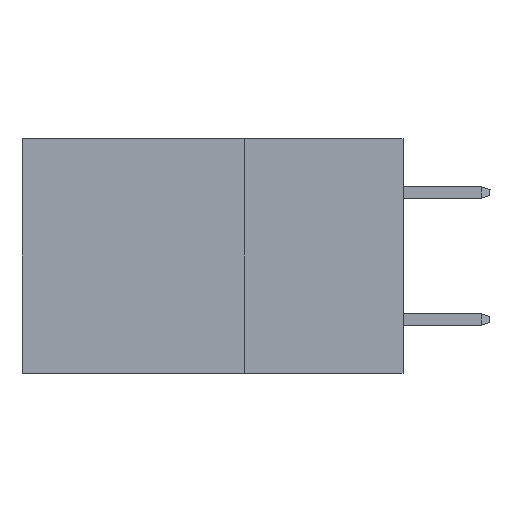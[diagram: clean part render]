
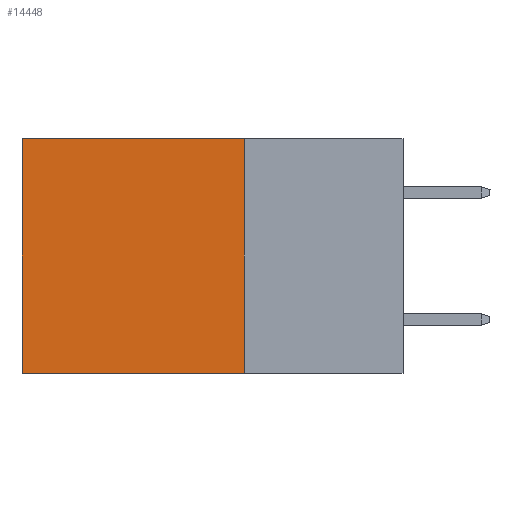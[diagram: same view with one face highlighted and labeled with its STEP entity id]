
A CAD part, left-side view. The second image highlights one B-rep face of the part: STEP entity #14448.
In plain terms, the highlighted planar face has unit normal (-1, 0, 0).
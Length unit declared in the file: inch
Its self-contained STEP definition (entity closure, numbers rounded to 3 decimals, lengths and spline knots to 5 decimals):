
#134 = DIRECTION ( 'NONE',  ( 0., 1., 0. ) ) ;
#319 = CARTESIAN_POINT ( 'NONE',  ( 0.2875, 0.6, 0. ) ) ;
#532 = PLANE ( 'NONE',  #3346 ) ;
#614 = FACE_OUTER_BOUND ( 'NONE', #8487, .T. ) ;
#944 = VERTEX_POINT ( 'NONE', #319 ) ;
#1567 = CARTESIAN_POINT ( 'NONE',  ( 0.2875, 0.25, 0. ) ) ;
#1646 = VERTEX_POINT ( 'NONE', #4934 ) ;
#2343 = EDGE_CURVE ( 'NONE', #9712, #6447, #3693, .T. ) ;
#2449 = ORIENTED_EDGE ( 'NONE', *, *, #6213, .T. ) ;
#2608 = CARTESIAN_POINT ( 'NONE',  ( 0.2875, 0.25, 0. ) ) ;
#3262 = VECTOR ( 'NONE', #4886, 39.37008 ) ;
#3346 = AXIS2_PLACEMENT_3D ( 'NONE', #14876, #4416, #5697 ) ;
#3693 = LINE ( 'NONE', #8888, #5870 ) ;
#4402 = EDGE_CURVE ( 'NONE', #944, #1646, #10922, .T. ) ;
#4416 = DIRECTION ( 'NONE',  ( 1., 0., 0. ) ) ;
#4886 = DIRECTION ( 'NONE',  ( 0., 1., 0. ) ) ;
#4934 = CARTESIAN_POINT ( 'NONE',  ( 0.2875, 0.6, -0.37 ) ) ;
#5075 = DIRECTION ( 'NONE',  ( 0., 0., -1. ) ) ;
#5697 = DIRECTION ( 'NONE',  ( 0., 0., -1. ) ) ;
#5870 = VECTOR ( 'NONE', #5075, 39.37008 ) ;
#5937 = VECTOR ( 'NONE', #134, 39.37008 ) ;
#6213 = EDGE_CURVE ( 'NONE', #9712, #944, #7868, .T. ) ;
#6447 = VERTEX_POINT ( 'NONE', #16330 ) ;
#7868 = LINE ( 'NONE', #1567, #5937 ) ;
#7979 = ORIENTED_EDGE ( 'NONE', *, *, #4402, .T. ) ;
#8185 = EDGE_CURVE ( 'NONE', #6447, #1646, #13883, .T. ) ;
#8441 = DIRECTION ( 'NONE',  ( 0., 0., -1. ) ) ;
#8487 = EDGE_LOOP ( 'NONE', ( #7979, #9019, #13822, #2449 ) ) ;
#8888 = CARTESIAN_POINT ( 'NONE',  ( 0.2875, 0.25, 0. ) ) ;
#9019 = ORIENTED_EDGE ( 'NONE', *, *, #8185, .F. ) ;
#9712 = VERTEX_POINT ( 'NONE', #2608 ) ;
#10922 = LINE ( 'NONE', #16016, #13524 ) ;
#13524 = VECTOR ( 'NONE', #8441, 39.37008 ) ;
#13822 = ORIENTED_EDGE ( 'NONE', *, *, #2343, .F. ) ;
#13883 = LINE ( 'NONE', #16528, #3262 ) ;
#14448 = ADVANCED_FACE ( 'NONE', ( #614 ), #532, .F. ) ;
#14876 = CARTESIAN_POINT ( 'NONE',  ( 0.2875, 0.25, 0. ) ) ;
#16016 = CARTESIAN_POINT ( 'NONE',  ( 0.2875, 0.6, 0. ) ) ;
#16330 = CARTESIAN_POINT ( 'NONE',  ( 0.2875, 0.25, -0.37 ) ) ;
#16528 = CARTESIAN_POINT ( 'NONE',  ( 0.2875, 0.25, -0.37 ) ) ;
